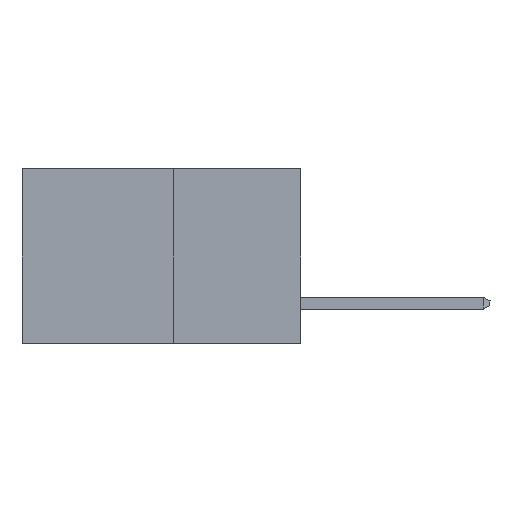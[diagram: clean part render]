
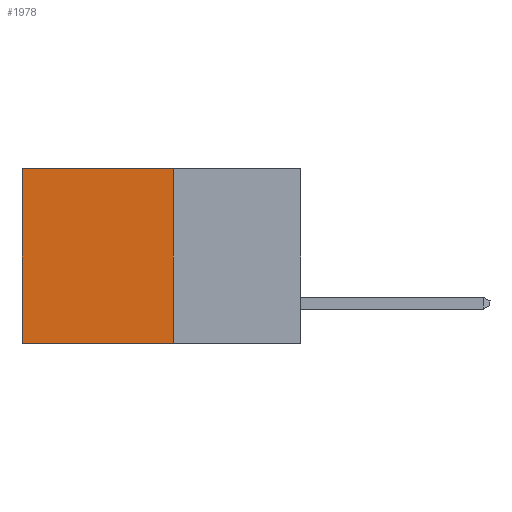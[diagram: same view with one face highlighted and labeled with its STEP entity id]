
A CAD part, left-side view. The second image highlights one B-rep face of the part: STEP entity #1978.
In plain terms, the highlighted planar face has unit normal (-1, 0, 0).
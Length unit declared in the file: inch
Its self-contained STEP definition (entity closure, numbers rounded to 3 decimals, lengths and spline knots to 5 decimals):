
#181 = DIRECTION ( 'NONE',  ( 0., 0., -1. ) ) ;
#344 = VECTOR ( 'NONE', #181, 39.37008 ) ;
#432 = EDGE_CURVE ( 'NONE', #6244, #5697, #2197, .T. ) ;
#515 = EDGE_CURVE ( 'NONE', #3119, #8973, #10094, .T. ) ;
#646 = AXIS2_PLACEMENT_3D ( 'NONE', #9975, #5377, #5162 ) ;
#1433 = DIRECTION ( 'NONE',  ( 0., 1., 0. ) ) ;
#1978 = ADVANCED_FACE ( 'NONE', ( #5469 ), #9985, .F. ) ;
#2197 = LINE ( 'NONE', #10091, #9168 ) ;
#2358 = EDGE_LOOP ( 'NONE', ( #4658, #11187, #7546, #11137 ) ) ;
#2828 = CARTESIAN_POINT ( 'NONE',  ( 0.277, 0.27, 0. ) ) ;
#2912 = LINE ( 'NONE', #9413, #344 ) ;
#2970 = EDGE_CURVE ( 'NONE', #8973, #5697, #9788, .T. ) ;
#3119 = VERTEX_POINT ( 'NONE', #4116 ) ;
#3913 = CARTESIAN_POINT ( 'NONE',  ( 0.277, 0.59, 0. ) ) ;
#4116 = CARTESIAN_POINT ( 'NONE',  ( 0.277, 0.27, 0. ) ) ;
#4658 = ORIENTED_EDGE ( 'NONE', *, *, #2970, .T. ) ;
#5005 = VECTOR ( 'NONE', #7657, 39.37008 ) ;
#5162 = DIRECTION ( 'NONE',  ( 0., 0., -1. ) ) ;
#5377 = DIRECTION ( 'NONE',  ( 1., 0., 0. ) ) ;
#5469 = FACE_OUTER_BOUND ( 'NONE', #2358, .T. ) ;
#5697 = VERTEX_POINT ( 'NONE', #6710 ) ;
#6244 = VERTEX_POINT ( 'NONE', #7777 ) ;
#6710 = CARTESIAN_POINT ( 'NONE',  ( 0.277, 0.59, -0.37 ) ) ;
#7335 = DIRECTION ( 'NONE',  ( 0., 1., 0. ) ) ;
#7480 = VECTOR ( 'NONE', #1433, 39.37008 ) ;
#7546 = ORIENTED_EDGE ( 'NONE', *, *, #9246, .F. ) ;
#7657 = DIRECTION ( 'NONE',  ( 0., 0., -1. ) ) ;
#7777 = CARTESIAN_POINT ( 'NONE',  ( 0.277, 0.27, -0.37 ) ) ;
#8443 = CARTESIAN_POINT ( 'NONE',  ( 0.277, 0.59, -0.37 ) ) ;
#8973 = VERTEX_POINT ( 'NONE', #3913 ) ;
#9168 = VECTOR ( 'NONE', #7335, 39.37008 ) ;
#9246 = EDGE_CURVE ( 'NONE', #3119, #6244, #2912, .T. ) ;
#9413 = CARTESIAN_POINT ( 'NONE',  ( 0.277, 0.27, -0.37 ) ) ;
#9788 = LINE ( 'NONE', #8443, #5005 ) ;
#9975 = CARTESIAN_POINT ( 'NONE',  ( 0.277, 0.27, -0.37 ) ) ;
#9985 = PLANE ( 'NONE',  #646 ) ;
#10091 = CARTESIAN_POINT ( 'NONE',  ( 0.277, 0.27, -0.37 ) ) ;
#10094 = LINE ( 'NONE', #2828, #7480 ) ;
#11137 = ORIENTED_EDGE ( 'NONE', *, *, #515, .T. ) ;
#11187 = ORIENTED_EDGE ( 'NONE', *, *, #432, .F. ) ;
